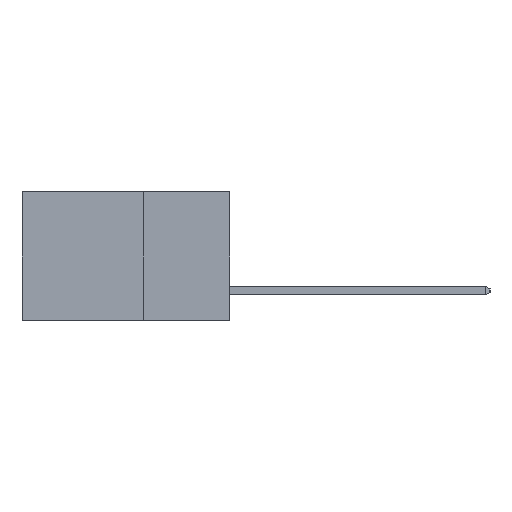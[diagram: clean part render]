
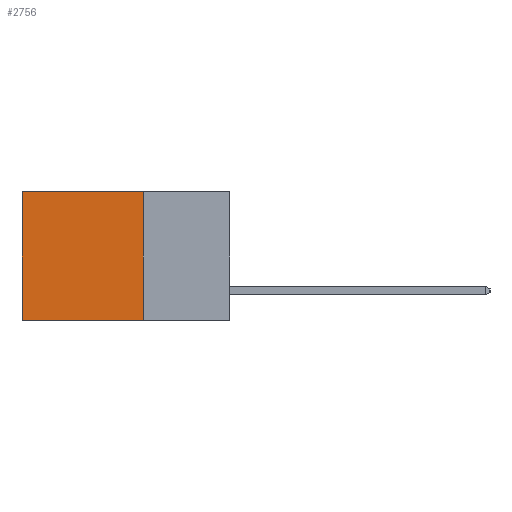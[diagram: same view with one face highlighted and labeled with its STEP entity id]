
A CAD part, left-side view. The second image highlights one B-rep face of the part: STEP entity #2756.
In plain terms, the highlighted planar face has unit normal (-1, 0, 0).
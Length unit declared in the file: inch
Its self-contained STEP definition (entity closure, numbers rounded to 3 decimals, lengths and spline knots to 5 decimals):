
#79 = LINE ( 'NONE', #999, #7907 ) ;
#654 = VERTEX_POINT ( 'NONE', #9613 ) ;
#822 = EDGE_CURVE ( 'NONE', #2984, #1210, #79, .T. ) ;
#999 = CARTESIAN_POINT ( 'NONE',  ( 0.2615, 0.6, -0.37 ) ) ;
#1089 = EDGE_CURVE ( 'NONE', #2409, #1210, #8166, .T. ) ;
#1210 = VERTEX_POINT ( 'NONE', #5343 ) ;
#1816 = EDGE_CURVE ( 'NONE', #654, #2984, #6770, .T. ) ;
#1819 = VECTOR ( 'NONE', #7927, 39.37008 ) ;
#2028 = DIRECTION ( 'NONE',  ( 0., 0., -1. ) ) ;
#2097 = DIRECTION ( 'NONE',  ( 1., 0., 0. ) ) ;
#2129 = CARTESIAN_POINT ( 'NONE',  ( 0.2615, 0.25, -0.37 ) ) ;
#2274 = EDGE_LOOP ( 'NONE', ( #5223, #2642, #8892, #2788 ) ) ;
#2333 = PLANE ( 'NONE',  #10613 ) ;
#2409 = VERTEX_POINT ( 'NONE', #10064 ) ;
#2523 = DIRECTION ( 'NONE',  ( 0., 0., -1. ) ) ;
#2642 = ORIENTED_EDGE ( 'NONE', *, *, #1089, .F. ) ;
#2756 = ADVANCED_FACE ( 'NONE', ( #7447 ), #2333, .F. ) ;
#2788 = ORIENTED_EDGE ( 'NONE', *, *, #1816, .T. ) ;
#2984 = VERTEX_POINT ( 'NONE', #11206 ) ;
#3386 = EDGE_CURVE ( 'NONE', #654, #2409, #12277, .T. ) ;
#3710 = DIRECTION ( 'NONE',  ( 0., 1., 0. ) ) ;
#3993 = CARTESIAN_POINT ( 'NONE',  ( 0.2615, 0.25, 0. ) ) ;
#4239 = DIRECTION ( 'NONE',  ( 0., 1., 0. ) ) ;
#5223 = ORIENTED_EDGE ( 'NONE', *, *, #822, .T. ) ;
#5343 = CARTESIAN_POINT ( 'NONE',  ( 0.2615, 0.6, -0.37 ) ) ;
#6770 = LINE ( 'NONE', #3993, #11358 ) ;
#7447 = FACE_OUTER_BOUND ( 'NONE', #2274, .T. ) ;
#7898 = VECTOR ( 'NONE', #3710, 39.37008 ) ;
#7907 = VECTOR ( 'NONE', #2523, 39.37008 ) ;
#7927 = DIRECTION ( 'NONE',  ( 0., 0., -1. ) ) ;
#7938 = CARTESIAN_POINT ( 'NONE',  ( 0.2615, 0.25, -0.37 ) ) ;
#8166 = LINE ( 'NONE', #10132, #7898 ) ;
#8892 = ORIENTED_EDGE ( 'NONE', *, *, #3386, .F. ) ;
#9613 = CARTESIAN_POINT ( 'NONE',  ( 0.2615, 0.25, 0. ) ) ;
#10064 = CARTESIAN_POINT ( 'NONE',  ( 0.2615, 0.25, -0.37 ) ) ;
#10132 = CARTESIAN_POINT ( 'NONE',  ( 0.2615, 0.25, -0.37 ) ) ;
#10613 = AXIS2_PLACEMENT_3D ( 'NONE', #2129, #2097, #2028 ) ;
#11206 = CARTESIAN_POINT ( 'NONE',  ( 0.2615, 0.6, 0. ) ) ;
#11358 = VECTOR ( 'NONE', #4239, 39.37008 ) ;
#12277 = LINE ( 'NONE', #7938, #1819 ) ;
